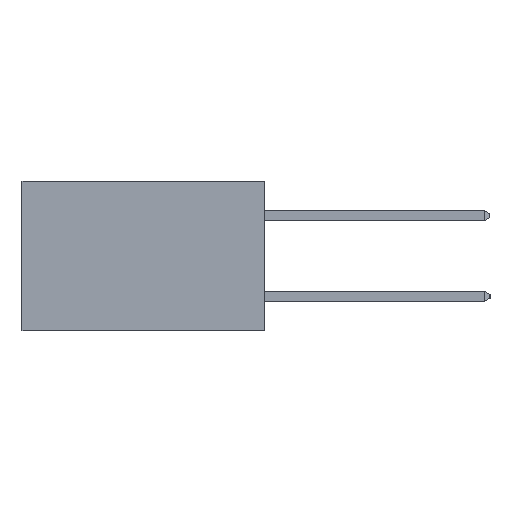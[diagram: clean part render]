
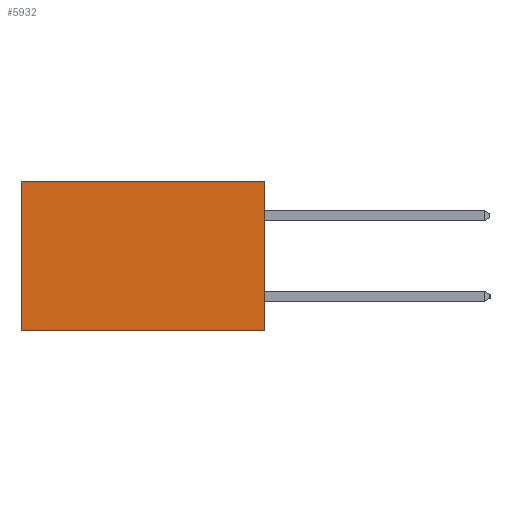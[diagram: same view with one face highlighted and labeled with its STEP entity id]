
A CAD part, left-side view. The second image highlights one B-rep face of the part: STEP entity #5932.
In plain terms, the highlighted planar face has unit normal (-1, 0, 0).
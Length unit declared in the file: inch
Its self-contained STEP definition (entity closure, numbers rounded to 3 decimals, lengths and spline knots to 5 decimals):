
#182 = DIRECTION ( 'NONE',  ( 0., 0., -1. ) ) ;
#278 = CARTESIAN_POINT ( 'NONE',  ( 0.2615, 0.6, 0. ) ) ;
#364 = VERTEX_POINT ( 'NONE', #19417 ) ;
#528 = CARTESIAN_POINT ( 'NONE',  ( 0.2615, 0., -0.37 ) ) ;
#1088 = CARTESIAN_POINT ( 'NONE',  ( 0.2615, 0., -0.37 ) ) ;
#1220 = FACE_OUTER_BOUND ( 'NONE', #9549, .T. ) ;
#1512 = LINE ( 'NONE', #1088, #2108 ) ;
#1687 = CARTESIAN_POINT ( 'NONE',  ( 0.2615, 0.6, -0.37 ) ) ;
#1768 = CARTESIAN_POINT ( 'NONE',  ( 0.2615, 0.6, -0.37 ) ) ;
#2108 = VECTOR ( 'NONE', #182, 39.37008 ) ;
#2720 = VECTOR ( 'NONE', #3619, 39.37008 ) ;
#3619 = DIRECTION ( 'NONE',  ( 0., 0., -1. ) ) ;
#3917 = ORIENTED_EDGE ( 'NONE', *, *, #5682, .F. ) ;
#4022 = LINE ( 'NONE', #528, #14103 ) ;
#4476 = AXIS2_PLACEMENT_3D ( 'NONE', #9167, #8831, #8539 ) ;
#4564 = VECTOR ( 'NONE', #15135, 39.37008 ) ;
#5682 = EDGE_CURVE ( 'NONE', #14148, #364, #1512, .T. ) ;
#5932 = ADVANCED_FACE ( 'NONE', ( #1220 ), #9558, .F. ) ;
#8539 = DIRECTION ( 'NONE',  ( 0., 0., -1. ) ) ;
#8831 = DIRECTION ( 'NONE',  ( 1., 0., 0. ) ) ;
#9167 = CARTESIAN_POINT ( 'NONE',  ( 0.2615, 0., -0.37 ) ) ;
#9472 = ORIENTED_EDGE ( 'NONE', *, *, #12302, .F. ) ;
#9549 = EDGE_LOOP ( 'NONE', ( #17633, #9472, #3917, #23984 ) ) ;
#9558 = PLANE ( 'NONE',  #4476 ) ;
#9985 = DIRECTION ( 'NONE',  ( 0., 1., 0. ) ) ;
#11395 = CARTESIAN_POINT ( 'NONE',  ( 0.2615, 0., 0. ) ) ;
#12302 = EDGE_CURVE ( 'NONE', #364, #17755, #4022, .T. ) ;
#14103 = VECTOR ( 'NONE', #9985, 39.37008 ) ;
#14148 = VERTEX_POINT ( 'NONE', #16233 ) ;
#15135 = DIRECTION ( 'NONE',  ( 0., 1., 0. ) ) ;
#16233 = CARTESIAN_POINT ( 'NONE',  ( 0.2615, 0., 0. ) ) ;
#17633 = ORIENTED_EDGE ( 'NONE', *, *, #23363, .T. ) ;
#17755 = VERTEX_POINT ( 'NONE', #1768 ) ;
#17844 = LINE ( 'NONE', #1687, #2720 ) ;
#18557 = VERTEX_POINT ( 'NONE', #278 ) ;
#19076 = EDGE_CURVE ( 'NONE', #14148, #18557, #19533, .T. ) ;
#19417 = CARTESIAN_POINT ( 'NONE',  ( 0.2615, 0., -0.37 ) ) ;
#19533 = LINE ( 'NONE', #11395, #4564 ) ;
#23363 = EDGE_CURVE ( 'NONE', #18557, #17755, #17844, .T. ) ;
#23984 = ORIENTED_EDGE ( 'NONE', *, *, #19076, .T. ) ;
